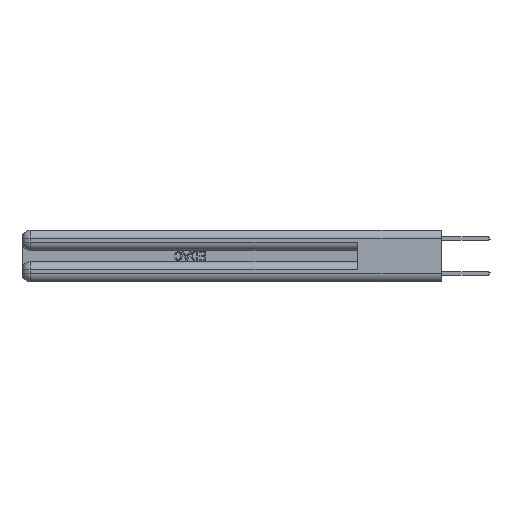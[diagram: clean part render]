
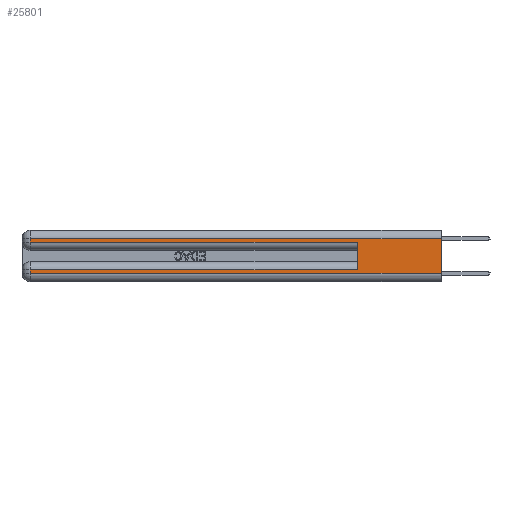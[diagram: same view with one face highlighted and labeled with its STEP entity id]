
A CAD part, left-side view. The second image highlights one B-rep face of the part: STEP entity #25801.
In plain terms, the highlighted planar face has unit normal (-1, 0, 0).
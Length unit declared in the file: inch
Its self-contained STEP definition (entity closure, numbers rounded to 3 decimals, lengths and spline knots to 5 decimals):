
#577 = EDGE_CURVE ( 'NONE', #16164, #14454, #23840, .T. ) ;
#1006 = VERTEX_POINT ( 'NONE', #2709 ) ;
#1093 = DIRECTION ( 'NONE',  ( 0., 0., -1. ) ) ;
#1207 = LINE ( 'NONE', #19930, #32657 ) ;
#2152 = VECTOR ( 'NONE', #20062, 39.37008 ) ;
#2398 = CARTESIAN_POINT ( 'NONE',  ( 0., 0., 0.285 ) ) ;
#2709 = CARTESIAN_POINT ( 'NONE',  ( 0., 0.6, 0.085 ) ) ;
#2836 = VECTOR ( 'NONE', #31812, 39.37008 ) ;
#2845 = DIRECTION ( 'NONE',  ( 0., 1., 0. ) ) ;
#3099 = VERTEX_POINT ( 'NONE', #6054 ) ;
#3165 = CARTESIAN_POINT ( 'NONE',  ( 0., 2.94, 0.37 ) ) ;
#3271 = AXIS2_PLACEMENT_3D ( 'NONE', #34324, #27624, #32722 ) ;
#3973 = EDGE_CURVE ( 'NONE', #1006, #16164, #11260, .T. ) ;
#4544 = EDGE_CURVE ( 'NONE', #3099, #19924, #8213, .T. ) ;
#5407 = EDGE_CURVE ( 'NONE', #17402, #11364, #17190, .T. ) ;
#5662 = CARTESIAN_POINT ( 'NONE',  ( 0., 0., 0.06 ) ) ;
#6053 = LINE ( 'NONE', #14464, #2152 ) ;
#6054 = CARTESIAN_POINT ( 'NONE',  ( 0., 0., 0.31 ) ) ;
#6165 = CARTESIAN_POINT ( 'NONE',  ( 0., 2.94, 0.37 ) ) ;
#6343 = VECTOR ( 'NONE', #1093, 39.37008 ) ;
#8213 = LINE ( 'NONE', #18564, #32059 ) ;
#8511 = VECTOR ( 'NONE', #2845, 39.37008 ) ;
#8721 = DIRECTION ( 'NONE',  ( 0., -1., 0. ) ) ;
#9079 = CARTESIAN_POINT ( 'NONE',  ( 0., 2.94, 0.085 ) ) ;
#9494 = VECTOR ( 'NONE', #22011, 39.37008 ) ;
#10485 = ORIENTED_EDGE ( 'NONE', *, *, #3973, .T. ) ;
#10535 = ORIENTED_EDGE ( 'NONE', *, *, #4544, .F. ) ;
#10803 = LINE ( 'NONE', #24608, #9494 ) ;
#11101 = EDGE_CURVE ( 'NONE', #14454, #19924, #1207, .T. ) ;
#11260 = LINE ( 'NONE', #29114, #8511 ) ;
#11319 = ORIENTED_EDGE ( 'NONE', *, *, #5407, .T. ) ;
#11364 = VERTEX_POINT ( 'NONE', #31829 ) ;
#11484 = EDGE_CURVE ( 'NONE', #1006, #21188, #6053, .T. ) ;
#12380 = VECTOR ( 'NONE', #26983, 39.37008 ) ;
#13503 = DIRECTION ( 'NONE',  ( 0., 0., -1. ) ) ;
#13600 = LINE ( 'NONE', #2398, #2836 ) ;
#14220 = CARTESIAN_POINT ( 'NONE',  ( 0., 2.94, 0.06 ) ) ;
#14454 = VERTEX_POINT ( 'NONE', #14220 ) ;
#14464 = CARTESIAN_POINT ( 'NONE',  ( 0., 0.6, 0.145 ) ) ;
#15917 = FACE_OUTER_BOUND ( 'NONE', #16832, .T. ) ;
#16164 = VERTEX_POINT ( 'NONE', #9079 ) ;
#16832 = EDGE_LOOP ( 'NONE', ( #10535, #22424, #11319, #34104, #31518, #10485, #29994, #16966 ) ) ;
#16966 = ORIENTED_EDGE ( 'NONE', *, *, #11101, .T. ) ;
#17190 = LINE ( 'NONE', #6165, #6343 ) ;
#17402 = VERTEX_POINT ( 'NONE', #17497 ) ;
#17497 = CARTESIAN_POINT ( 'NONE',  ( 0., 2.94, 0.31 ) ) ;
#18564 = CARTESIAN_POINT ( 'NONE',  ( 0., 0., 0.37 ) ) ;
#19382 = EDGE_CURVE ( 'NONE', #11364, #21188, #13600, .T. ) ;
#19924 = VERTEX_POINT ( 'NONE', #5662 ) ;
#19930 = CARTESIAN_POINT ( 'NONE',  ( 0., 0., 0.06 ) ) ;
#20062 = DIRECTION ( 'NONE',  ( 0., 0., 1. ) ) ;
#21188 = VERTEX_POINT ( 'NONE', #24411 ) ;
#22011 = DIRECTION ( 'NONE',  ( 0., 1., 0. ) ) ;
#22424 = ORIENTED_EDGE ( 'NONE', *, *, #26237, .T. ) ;
#23840 = LINE ( 'NONE', #3165, #12380 ) ;
#24411 = CARTESIAN_POINT ( 'NONE',  ( 0., 0.6, 0.285 ) ) ;
#24608 = CARTESIAN_POINT ( 'NONE',  ( 0., 0., 0.31 ) ) ;
#25801 = ADVANCED_FACE ( 'NONE', ( #15917 ), #28701, .F. ) ;
#26237 = EDGE_CURVE ( 'NONE', #3099, #17402, #10803, .T. ) ;
#26983 = DIRECTION ( 'NONE',  ( 0., 0., -1. ) ) ;
#27624 = DIRECTION ( 'NONE',  ( 1., 0., 0. ) ) ;
#28701 = PLANE ( 'NONE',  #3271 ) ;
#29114 = CARTESIAN_POINT ( 'NONE',  ( 0., 0., 0.085 ) ) ;
#29994 = ORIENTED_EDGE ( 'NONE', *, *, #577, .T. ) ;
#31518 = ORIENTED_EDGE ( 'NONE', *, *, #11484, .F. ) ;
#31812 = DIRECTION ( 'NONE',  ( 0., -1., 0. ) ) ;
#31829 = CARTESIAN_POINT ( 'NONE',  ( 0., 2.94, 0.285 ) ) ;
#32059 = VECTOR ( 'NONE', #13503, 39.37008 ) ;
#32657 = VECTOR ( 'NONE', #8721, 39.37008 ) ;
#32722 = DIRECTION ( 'NONE',  ( 0., 0., -1. ) ) ;
#34104 = ORIENTED_EDGE ( 'NONE', *, *, #19382, .T. ) ;
#34324 = CARTESIAN_POINT ( 'NONE',  ( 0., 0., 0.37 ) ) ;
